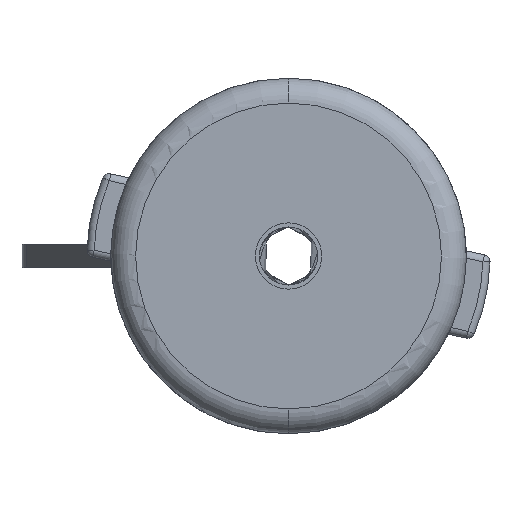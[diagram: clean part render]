
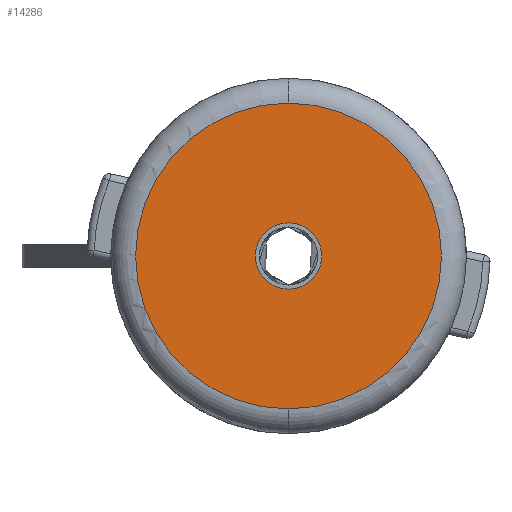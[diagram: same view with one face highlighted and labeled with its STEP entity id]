
A CAD part, front view. The second image highlights one B-rep face of the part: STEP entity #14286.
In plain terms, the highlighted planar face has unit normal (0, -1, 0).
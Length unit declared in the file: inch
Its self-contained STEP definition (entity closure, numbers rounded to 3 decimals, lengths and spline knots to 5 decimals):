
#442 = AXIS2_PLACEMENT_3D ( 'NONE', #2912, #11186, #4110 ) ;
#577 = CARTESIAN_POINT ( 'NONE',  ( 0., 0., -0.14 ) ) ;
#1221 = CIRCLE ( 'NONE', #442, 0.14 ) ;
#1329 = CARTESIAN_POINT ( 'NONE',  ( 0., 0., 0. ) ) ;
#1602 = CARTESIAN_POINT ( 'NONE',  ( 0., 0., 0. ) ) ;
#2159 = AXIS2_PLACEMENT_3D ( 'NONE', #1329, #6293, #14569 ) ;
#2823 = DIRECTION ( 'NONE',  ( 0., 0., -1. ) ) ;
#2912 = CARTESIAN_POINT ( 'NONE',  ( 0., 0., 0. ) ) ;
#3055 = EDGE_LOOP ( 'NONE', ( #3086, #9907 ) ) ;
#3086 = ORIENTED_EDGE ( 'NONE', *, *, #8558, .T. ) ;
#3509 = DIRECTION ( 'NONE',  ( 0., -1., 0. ) ) ;
#3566 = VERTEX_POINT ( 'NONE', #14380 ) ;
#4110 = DIRECTION ( 'NONE',  ( 0., 0., 1. ) ) ;
#4312 = CIRCLE ( 'NONE', #6816, 0.645 ) ;
#5179 = EDGE_CURVE ( 'NONE', #9713, #13782, #5628, .T. ) ;
#5628 = CIRCLE ( 'NONE', #5816, 0.14 ) ;
#5816 = AXIS2_PLACEMENT_3D ( 'NONE', #7044, #15301, #8214 ) ;
#6293 = DIRECTION ( 'NONE',  ( 0., -1., 0. ) ) ;
#6688 = EDGE_CURVE ( 'NONE', #3566, #14720, #4312, .T. ) ;
#6816 = AXIS2_PLACEMENT_3D ( 'NONE', #10579, #3509, #11791 ) ;
#7044 = CARTESIAN_POINT ( 'NONE',  ( 0., 0., 0. ) ) ;
#8214 = DIRECTION ( 'NONE',  ( 0., 0., 1. ) ) ;
#8348 = EDGE_LOOP ( 'NONE', ( #13971, #11206 ) ) ;
#8558 = EDGE_CURVE ( 'NONE', #14720, #3566, #9501, .T. ) ;
#9501 = CIRCLE ( 'NONE', #14642, 0.645 ) ;
#9713 = VERTEX_POINT ( 'NONE', #577 ) ;
#9744 = FACE_BOUND ( 'NONE', #8348, .T. ) ;
#9907 = ORIENTED_EDGE ( 'NONE', *, *, #6688, .T. ) ;
#9922 = DIRECTION ( 'NONE',  ( 0., -1., 0. ) ) ;
#10579 = CARTESIAN_POINT ( 'NONE',  ( 0., 0., 0. ) ) ;
#11132 = EDGE_CURVE ( 'NONE', #13782, #9713, #1221, .T. ) ;
#11186 = DIRECTION ( 'NONE',  ( 0., 1., 0. ) ) ;
#11206 = ORIENTED_EDGE ( 'NONE', *, *, #11132, .T. ) ;
#11791 = DIRECTION ( 'NONE',  ( 0., 0., -1. ) ) ;
#12922 = FACE_OUTER_BOUND ( 'NONE', #3055, .T. ) ;
#13231 = CARTESIAN_POINT ( 'NONE',  ( 0., 0., -0.645 ) ) ;
#13371 = PLANE ( 'NONE',  #2159 ) ;
#13782 = VERTEX_POINT ( 'NONE', #15006 ) ;
#13971 = ORIENTED_EDGE ( 'NONE', *, *, #5179, .T. ) ;
#14286 = ADVANCED_FACE ( 'NONE', ( #12922, #9744 ), #13371, .T. ) ;
#14380 = CARTESIAN_POINT ( 'NONE',  ( 0., 0., 0.645 ) ) ;
#14569 = DIRECTION ( 'NONE',  ( 0., 0., -1. ) ) ;
#14642 = AXIS2_PLACEMENT_3D ( 'NONE', #1602, #9922, #2823 ) ;
#14720 = VERTEX_POINT ( 'NONE', #13231 ) ;
#15006 = CARTESIAN_POINT ( 'NONE',  ( 0., 0., 0.14 ) ) ;
#15301 = DIRECTION ( 'NONE',  ( 0., 1., 0. ) ) ;
